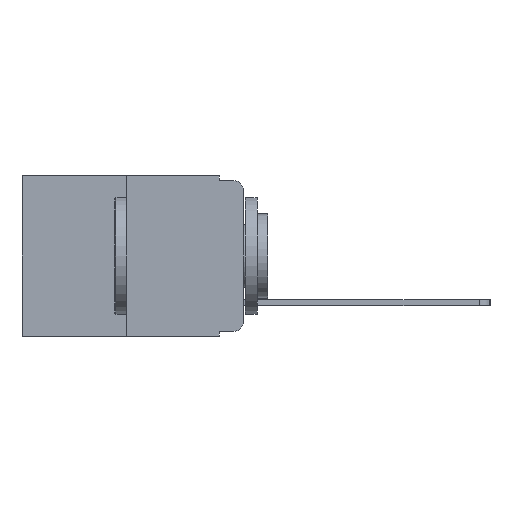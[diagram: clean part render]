
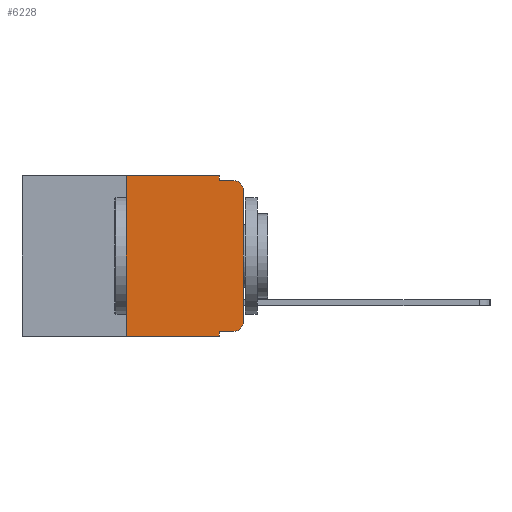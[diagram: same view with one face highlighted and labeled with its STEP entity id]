
A CAD part, left-side view. The second image highlights one B-rep face of the part: STEP entity #6228.
In plain terms, the highlighted planar face has unit normal (-1, 0, 0).
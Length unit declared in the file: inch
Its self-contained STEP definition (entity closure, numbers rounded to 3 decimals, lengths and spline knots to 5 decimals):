
#28 = EDGE_CURVE ( 'NONE', #3026, #12306, #12186, .T. ) ;
#57 = EDGE_LOOP ( 'NONE', ( #6350, #8677, #2275, #5384, #8830, #2440, #8368, #487, #6908, #2614 ) ) ;
#69 = LINE ( 'NONE', #11430, #5503 ) ;
#286 = DIRECTION ( 'NONE',  ( 0., 0., -1. ) ) ;
#468 = VERTEX_POINT ( 'NONE', #4586 ) ;
#487 = ORIENTED_EDGE ( 'NONE', *, *, #3055, .F. ) ;
#798 = EDGE_CURVE ( 'NONE', #6873, #3026, #9462, .T. ) ;
#986 = CARTESIAN_POINT ( 'NONE',  ( 0., 0.25, -0.343 ) ) ;
#1082 = CARTESIAN_POINT ( 'NONE',  ( 0., 0., -0.03 ) ) ;
#1451 = CARTESIAN_POINT ( 'NONE',  ( 0., 0.25, 0. ) ) ;
#1460 = DIRECTION ( 'NONE',  ( 0., 0., 1. ) ) ;
#1462 = FACE_OUTER_BOUND ( 'NONE', #57, .T. ) ;
#1513 = AXIS2_PLACEMENT_3D ( 'NONE', #12737, #2016, #2031 ) ;
#1598 = VECTOR ( 'NONE', #12066, 39.37008 ) ;
#1821 = CARTESIAN_POINT ( 'NONE',  ( 0., 0.051, 0. ) ) ;
#2016 = DIRECTION ( 'NONE',  ( -1., 0., 0. ) ) ;
#2031 = DIRECTION ( 'NONE',  ( 0., 0., -1. ) ) ;
#2162 = CARTESIAN_POINT ( 'NONE',  ( 0., 0.02, -0.03 ) ) ;
#2275 = ORIENTED_EDGE ( 'NONE', *, *, #6541, .F. ) ;
#2440 = ORIENTED_EDGE ( 'NONE', *, *, #4442, .F. ) ;
#2614 = ORIENTED_EDGE ( 'NONE', *, *, #28, .T. ) ;
#2640 = CARTESIAN_POINT ( 'NONE',  ( 0., 0.25, 0. ) ) ;
#2790 = CARTESIAN_POINT ( 'NONE',  ( 0., 0.051, -0.333 ) ) ;
#2811 = VERTEX_POINT ( 'NONE', #4898 ) ;
#3000 = LINE ( 'NONE', #1821, #1598 ) ;
#3026 = VERTEX_POINT ( 'NONE', #12639 ) ;
#3055 = EDGE_CURVE ( 'NONE', #6873, #468, #69, .T. ) ;
#3242 = DIRECTION ( 'NONE',  ( 0., 0., -1. ) ) ;
#3367 = CARTESIAN_POINT ( 'NONE',  ( 0., 0., -0.313 ) ) ;
#3632 = LINE ( 'NONE', #5968, #11449 ) ;
#4141 = LINE ( 'NONE', #6152, #6579 ) ;
#4411 = VECTOR ( 'NONE', #11431, 39.37008 ) ;
#4442 = EDGE_CURVE ( 'NONE', #10351, #7499, #9676, .T. ) ;
#4586 = CARTESIAN_POINT ( 'NONE',  ( 0., 0.051, -0.343 ) ) ;
#4629 = PLANE ( 'NONE',  #4696 ) ;
#4696 = AXIS2_PLACEMENT_3D ( 'NONE', #10775, #6756, #286 ) ;
#4898 = CARTESIAN_POINT ( 'NONE',  ( 0., 0.051, 0. ) ) ;
#4915 = CARTESIAN_POINT ( 'NONE',  ( 0., 0.051, -0.01 ) ) ;
#5318 = EDGE_CURVE ( 'NONE', #10351, #468, #4141, .T. ) ;
#5351 = CARTESIAN_POINT ( 'NONE',  ( 0., 0., 0. ) ) ;
#5384 = ORIENTED_EDGE ( 'NONE', *, *, #5845, .F. ) ;
#5503 = VECTOR ( 'NONE', #9052, 39.37008 ) ;
#5845 = EDGE_CURVE ( 'NONE', #2811, #11414, #3000, .T. ) ;
#5968 = CARTESIAN_POINT ( 'NONE',  ( 0., 0.473, 0. ) ) ;
#6152 = CARTESIAN_POINT ( 'NONE',  ( 0., 0.473, -0.343 ) ) ;
#6228 = ADVANCED_FACE ( 'NONE', ( #1462 ), #4629, .F. ) ;
#6350 = ORIENTED_EDGE ( 'NONE', *, *, #8669, .T. ) ;
#6541 = EDGE_CURVE ( 'NONE', #11414, #7426, #9041, .T. ) ;
#6579 = VECTOR ( 'NONE', #7343, 39.37008 ) ;
#6600 = VECTOR ( 'NONE', #9490, 39.37008 ) ;
#6756 = DIRECTION ( 'NONE',  ( 1., 0., 0. ) ) ;
#6873 = VERTEX_POINT ( 'NONE', #6897 ) ;
#6897 = CARTESIAN_POINT ( 'NONE',  ( 0., 0.051, -0.333 ) ) ;
#6908 = ORIENTED_EDGE ( 'NONE', *, *, #798, .T. ) ;
#7242 = VERTEX_POINT ( 'NONE', #1082 ) ;
#7343 = DIRECTION ( 'NONE',  ( 0., -1., 0. ) ) ;
#7426 = VERTEX_POINT ( 'NONE', #10701 ) ;
#7499 = VERTEX_POINT ( 'NONE', #2640 ) ;
#7649 = EDGE_CURVE ( 'NONE', #7499, #2811, #3632, .T. ) ;
#7997 = EDGE_CURVE ( 'NONE', #7242, #7426, #10069, .T. ) ;
#8163 = DIRECTION ( 'NONE',  ( 0., -1., 0. ) ) ;
#8368 = ORIENTED_EDGE ( 'NONE', *, *, #5318, .T. ) ;
#8496 = CARTESIAN_POINT ( 'NONE',  ( 0., 0.051, -0.01 ) ) ;
#8669 = EDGE_CURVE ( 'NONE', #12306, #7242, #12156, .T. ) ;
#8677 = ORIENTED_EDGE ( 'NONE', *, *, #7997, .T. ) ;
#8830 = ORIENTED_EDGE ( 'NONE', *, *, #7649, .F. ) ;
#8997 = AXIS2_PLACEMENT_3D ( 'NONE', #2162, #9456, #3242 ) ;
#9041 = LINE ( 'NONE', #8496, #6600 ) ;
#9052 = DIRECTION ( 'NONE',  ( 0., 0., -1. ) ) ;
#9159 = DIRECTION ( 'NONE',  ( 0., -1., 0. ) ) ;
#9456 = DIRECTION ( 'NONE',  ( -1., 0., 0. ) ) ;
#9462 = LINE ( 'NONE', #2790, #11429 ) ;
#9490 = DIRECTION ( 'NONE',  ( 0., -1., 0. ) ) ;
#9676 = LINE ( 'NONE', #1451, #10262 ) ;
#10069 = CIRCLE ( 'NONE', #8997, 0.02 ) ;
#10262 = VECTOR ( 'NONE', #1460, 39.37008 ) ;
#10351 = VERTEX_POINT ( 'NONE', #986 ) ;
#10701 = CARTESIAN_POINT ( 'NONE',  ( 0., 0.02, -0.01 ) ) ;
#10775 = CARTESIAN_POINT ( 'NONE',  ( 0., 0.473, 0. ) ) ;
#11414 = VERTEX_POINT ( 'NONE', #4915 ) ;
#11429 = VECTOR ( 'NONE', #8163, 39.37008 ) ;
#11430 = CARTESIAN_POINT ( 'NONE',  ( 0., 0.051, 0. ) ) ;
#11431 = DIRECTION ( 'NONE',  ( 0., 0., 1. ) ) ;
#11449 = VECTOR ( 'NONE', #9159, 39.37008 ) ;
#12066 = DIRECTION ( 'NONE',  ( 0., 0., -1. ) ) ;
#12156 = LINE ( 'NONE', #5351, #4411 ) ;
#12186 = CIRCLE ( 'NONE', #1513, 0.02 ) ;
#12306 = VERTEX_POINT ( 'NONE', #3367 ) ;
#12639 = CARTESIAN_POINT ( 'NONE',  ( 0., 0.02, -0.333 ) ) ;
#12737 = CARTESIAN_POINT ( 'NONE',  ( 0., 0.02, -0.313 ) ) ;
